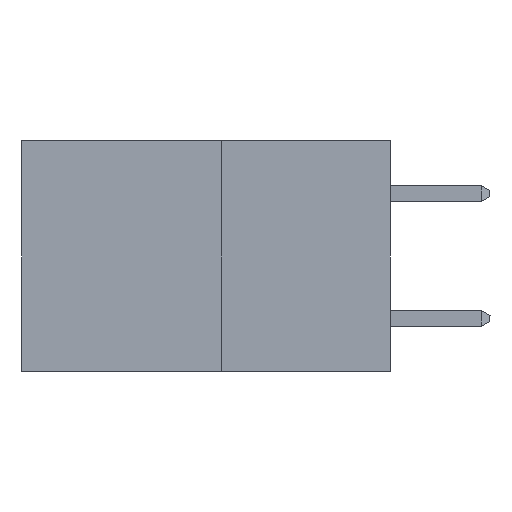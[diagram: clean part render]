
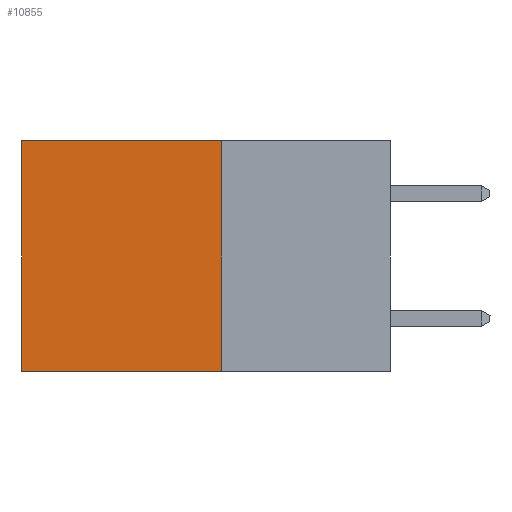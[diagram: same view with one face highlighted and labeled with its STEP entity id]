
A CAD part, left-side view. The second image highlights one B-rep face of the part: STEP entity #10855.
In plain terms, the highlighted planar face has unit normal (-1, 0, 0).
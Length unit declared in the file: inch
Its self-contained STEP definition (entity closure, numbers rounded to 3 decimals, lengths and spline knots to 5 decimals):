
#203 = ORIENTED_EDGE ( 'NONE', *, *, #12087, .T. ) ;
#2938 = VECTOR ( 'NONE', #19662, 39.37008 ) ;
#5169 = CARTESIAN_POINT ( 'NONE',  ( 0.277, 0.27, -0.37 ) ) ;
#5255 = EDGE_LOOP ( 'NONE', ( #14845, #7356, #12881, #203 ) ) ;
#6925 = EDGE_CURVE ( 'NONE', #14703, #24456, #12598, .T. ) ;
#7356 = ORIENTED_EDGE ( 'NONE', *, *, #6925, .F. ) ;
#7419 = VECTOR ( 'NONE', #18248, 39.37008 ) ;
#7777 = VERTEX_POINT ( 'NONE', #25072 ) ;
#7943 = DIRECTION ( 'NONE',  ( 0., 1., 0. ) ) ;
#8575 = VECTOR ( 'NONE', #7943, 39.37008 ) ;
#8681 = CARTESIAN_POINT ( 'NONE',  ( 0.277, 0.27, -0.37 ) ) ;
#8766 = LINE ( 'NONE', #13128, #2938 ) ;
#10354 = FACE_OUTER_BOUND ( 'NONE', #5255, .T. ) ;
#10855 = ADVANCED_FACE ( 'NONE', ( #10354 ), #19521, .F. ) ;
#10881 = DIRECTION ( 'NONE',  ( 0., 0., -1. ) ) ;
#12087 = EDGE_CURVE ( 'NONE', #7777, #25408, #15098, .T. ) ;
#12598 = LINE ( 'NONE', #5169, #7419 ) ;
#12881 = ORIENTED_EDGE ( 'NONE', *, *, #23412, .F. ) ;
#13128 = CARTESIAN_POINT ( 'NONE',  ( 0.277, 0.27, -0.37 ) ) ;
#13301 = AXIS2_PLACEMENT_3D ( 'NONE', #8681, #23860, #10881 ) ;
#14703 = VERTEX_POINT ( 'NONE', #22903 ) ;
#14845 = ORIENTED_EDGE ( 'NONE', *, *, #24125, .T. ) ;
#15098 = LINE ( 'NONE', #18816, #8575 ) ;
#17938 = DIRECTION ( 'NONE',  ( 0., 0., -1. ) ) ;
#18248 = DIRECTION ( 'NONE',  ( 0., 1., 0. ) ) ;
#18816 = CARTESIAN_POINT ( 'NONE',  ( 0.277, 0.27, 0. ) ) ;
#19521 = PLANE ( 'NONE',  #13301 ) ;
#19662 = DIRECTION ( 'NONE',  ( 0., 0., -1. ) ) ;
#19950 = LINE ( 'NONE', #20104, #24331 ) ;
#20104 = CARTESIAN_POINT ( 'NONE',  ( 0.277, 0.59, -0.37 ) ) ;
#21123 = CARTESIAN_POINT ( 'NONE',  ( 0.277, 0.59, -0.37 ) ) ;
#22903 = CARTESIAN_POINT ( 'NONE',  ( 0.277, 0.27, -0.37 ) ) ;
#23412 = EDGE_CURVE ( 'NONE', #7777, #14703, #8766, .T. ) ;
#23860 = DIRECTION ( 'NONE',  ( 1., 0., 0. ) ) ;
#24125 = EDGE_CURVE ( 'NONE', #25408, #24456, #19950, .T. ) ;
#24331 = VECTOR ( 'NONE', #17938, 39.37008 ) ;
#24456 = VERTEX_POINT ( 'NONE', #21123 ) ;
#25072 = CARTESIAN_POINT ( 'NONE',  ( 0.277, 0.27, 0. ) ) ;
#25408 = VERTEX_POINT ( 'NONE', #28004 ) ;
#28004 = CARTESIAN_POINT ( 'NONE',  ( 0.277, 0.59, 0. ) ) ;
